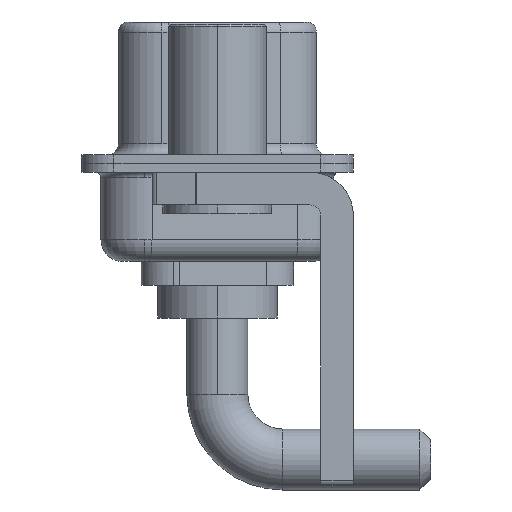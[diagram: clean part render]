
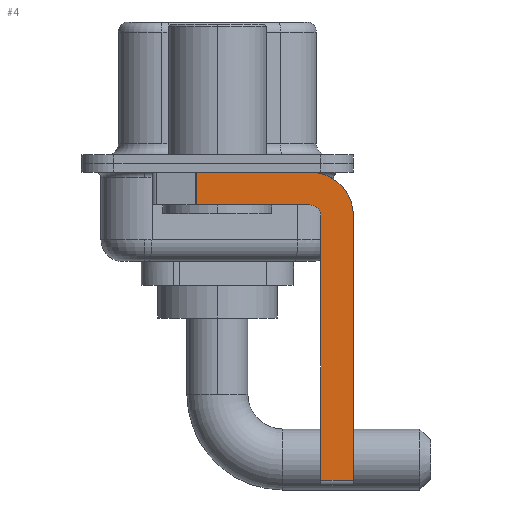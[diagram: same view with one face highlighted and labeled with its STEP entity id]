
A CAD part, left-side view. The second image highlights one B-rep face of the part: STEP entity #4.
In plain terms, the highlighted planar face has unit normal (-1, 0, 0).
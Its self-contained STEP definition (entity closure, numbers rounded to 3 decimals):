
#4 = ADVANCED_FACE ( 'NONE', ( #4116 ), #9720, .F. ) ;
#524 = CARTESIAN_POINT ( 'NONE',  ( -2.9, -4.75, -14.55 ) ) ;
#622 = CIRCLE ( 'NONE', #7109, 0.5 ) ;
#736 = CARTESIAN_POINT ( 'NONE',  ( -2.9, 0.978, -1.9 ) ) ;
#881 = VECTOR ( 'NONE', #7307, 1000. ) ;
#1029 = VERTEX_POINT ( 'NONE', #736 ) ;
#1038 = DIRECTION ( 'NONE',  ( 1., 0., 0. ) ) ;
#1373 = EDGE_CURVE ( 'NONE', #2605, #1029, #8886, .T. ) ;
#1557 = ORIENTED_EDGE ( 'NONE', *, *, #9559, .T. ) ;
#1759 = ORIENTED_EDGE ( 'NONE', *, *, #10866, .F. ) ;
#1877 = VERTEX_POINT ( 'NONE', #11922 ) ;
#1912 = CARTESIAN_POINT ( 'NONE',  ( -2.9, 0.978, -1.9 ) ) ;
#1983 = ORIENTED_EDGE ( 'NONE', *, *, #10088, .F. ) ;
#2605 = VERTEX_POINT ( 'NONE', #12607 ) ;
#2966 = LINE ( 'NONE', #16690, #12789 ) ;
#3220 = CARTESIAN_POINT ( 'NONE',  ( -2.9, -4.75, -14.8 ) ) ;
#3922 = EDGE_CURVE ( 'NONE', #6451, #7548, #2966, .T. ) ;
#4116 = FACE_OUTER_BOUND ( 'NONE', #11576, .T. ) ;
#4430 = ORIENTED_EDGE ( 'NONE', *, *, #1373, .T. ) ;
#4655 = DIRECTION ( 'NONE',  ( 0., 0., 1. ) ) ;
#5947 = CARTESIAN_POINT ( 'NONE',  ( -2.9, -4.25, -1.9 ) ) ;
#6143 = DIRECTION ( 'NONE',  ( 0., 0., 1. ) ) ;
#6451 = VERTEX_POINT ( 'NONE', #7516 ) ;
#7109 = AXIS2_PLACEMENT_3D ( 'NONE', #15950, #11649, #4655 ) ;
#7307 = DIRECTION ( 'NONE',  ( 0., -1., 0. ) ) ;
#7516 = CARTESIAN_POINT ( 'NONE',  ( -2.9, -6.25, -2.4 ) ) ;
#7548 = VERTEX_POINT ( 'NONE', #7563 ) ;
#7563 = CARTESIAN_POINT ( 'NONE',  ( -2.9, -6.25, -14.55 ) ) ;
#8523 = VECTOR ( 'NONE', #17278, 1000. ) ;
#8781 = AXIS2_PLACEMENT_3D ( 'NONE', #12654, #12299, #16438 ) ;
#8886 = LINE ( 'NONE', #1912, #8523 ) ;
#9201 = ORIENTED_EDGE ( 'NONE', *, *, #3922, .F. ) ;
#9559 = EDGE_CURVE ( 'NONE', #16111, #7548, #12569, .T. ) ;
#9645 = EDGE_CURVE ( 'NONE', #2605, #9805, #17061, .T. ) ;
#9720 = PLANE ( 'NONE',  #8781 ) ;
#9805 = VERTEX_POINT ( 'NONE', #12044 ) ;
#10088 = EDGE_CURVE ( 'NONE', #10778, #1029, #11668, .T. ) ;
#10273 = ORIENTED_EDGE ( 'NONE', *, *, #10625, .F. ) ;
#10340 = CIRCLE ( 'NONE', #11237, 2. ) ;
#10625 = EDGE_CURVE ( 'NONE', #1877, #10778, #622, .T. ) ;
#10778 = VERTEX_POINT ( 'NONE', #12366 ) ;
#10866 = EDGE_CURVE ( 'NONE', #9805, #6451, #10340, .T. ) ;
#11237 = AXIS2_PLACEMENT_3D ( 'NONE', #16510, #1038, #15388 ) ;
#11371 = CARTESIAN_POINT ( 'NONE',  ( -2.9, 3., -0.4 ) ) ;
#11576 = EDGE_LOOP ( 'NONE', ( #13765, #4430, #1983, #10273, #15589, #1557, #9201, #1759 ) ) ;
#11649 = DIRECTION ( 'NONE',  ( -1., 0., 0. ) ) ;
#11668 = LINE ( 'NONE', #5947, #12074 ) ;
#11922 = CARTESIAN_POINT ( 'NONE',  ( -2.9, -4.75, -2.4 ) ) ;
#12044 = CARTESIAN_POINT ( 'NONE',  ( -2.9, -4.25, -0.4 ) ) ;
#12074 = VECTOR ( 'NONE', #13122, 1000. ) ;
#12296 = CARTESIAN_POINT ( 'NONE',  ( -2.9, -4.25, -14.55 ) ) ;
#12299 = DIRECTION ( 'NONE',  ( 1., 0., 0. ) ) ;
#12366 = CARTESIAN_POINT ( 'NONE',  ( -2.9, -4.25, -1.9 ) ) ;
#12569 = LINE ( 'NONE', #12296, #16173 ) ;
#12607 = CARTESIAN_POINT ( 'NONE',  ( -2.9, 0.978, -0.4 ) ) ;
#12654 = CARTESIAN_POINT ( 'NONE',  ( -2.9, -4.25, -2.4 ) ) ;
#12789 = VECTOR ( 'NONE', #15206, 1000. ) ;
#13122 = DIRECTION ( 'NONE',  ( 0., 1., 0. ) ) ;
#13253 = VECTOR ( 'NONE', #6143, 1000. ) ;
#13765 = ORIENTED_EDGE ( 'NONE', *, *, #9645, .F. ) ;
#14432 = LINE ( 'NONE', #3220, #13253 ) ;
#15206 = DIRECTION ( 'NONE',  ( 0., 0., -1. ) ) ;
#15388 = DIRECTION ( 'NONE',  ( 0., 0., -1. ) ) ;
#15589 = ORIENTED_EDGE ( 'NONE', *, *, #15635, .F. ) ;
#15635 = EDGE_CURVE ( 'NONE', #16111, #1877, #14432, .T. ) ;
#15950 = CARTESIAN_POINT ( 'NONE',  ( -2.9, -4.25, -2.4 ) ) ;
#16111 = VERTEX_POINT ( 'NONE', #524 ) ;
#16173 = VECTOR ( 'NONE', #18076, 1000. ) ;
#16438 = DIRECTION ( 'NONE',  ( 0., 0., -1. ) ) ;
#16510 = CARTESIAN_POINT ( 'NONE',  ( -2.9, -4.25, -2.4 ) ) ;
#16690 = CARTESIAN_POINT ( 'NONE',  ( -2.9, -6.25, -2.4 ) ) ;
#17061 = LINE ( 'NONE', #11371, #881 ) ;
#17278 = DIRECTION ( 'NONE',  ( 0., 0., -1. ) ) ;
#18076 = DIRECTION ( 'NONE',  ( 0., -1., 0. ) ) ;
